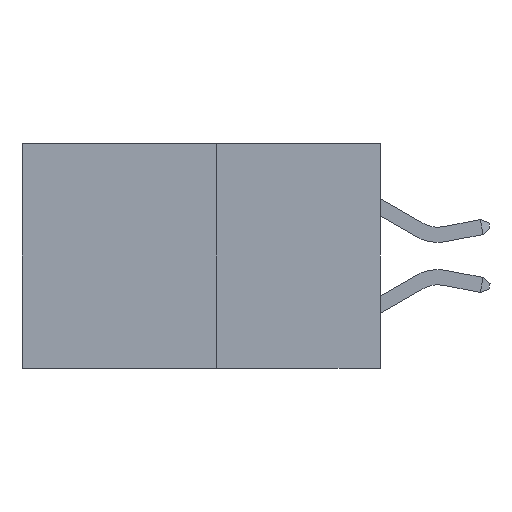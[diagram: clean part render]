
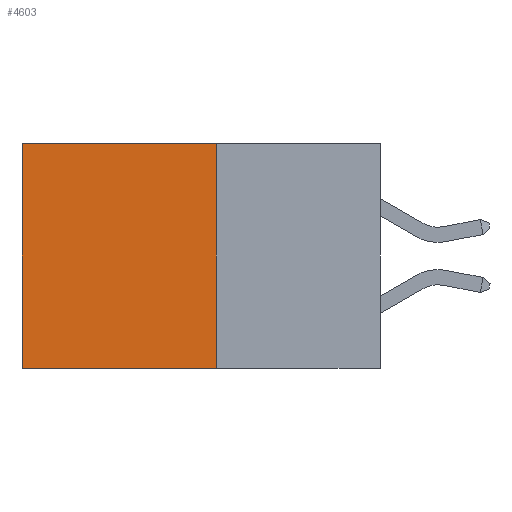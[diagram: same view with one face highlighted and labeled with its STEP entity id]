
A CAD part, left-side view. The second image highlights one B-rep face of the part: STEP entity #4603.
In plain terms, the highlighted planar face has unit normal (-1, 0, 0).
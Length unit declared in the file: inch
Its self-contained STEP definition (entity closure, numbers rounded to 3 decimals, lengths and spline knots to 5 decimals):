
#273 = FACE_OUTER_BOUND ( 'NONE', #3999, .T. ) ;
#633 = ORIENTED_EDGE ( 'NONE', *, *, #11598, .T. ) ;
#1055 = CARTESIAN_POINT ( 'NONE',  ( 0.277, 0.59, -0.37 ) ) ;
#1061 = LINE ( 'NONE', #1055, #3337 ) ;
#1220 = DIRECTION ( 'NONE',  ( 0., 1., 0. ) ) ;
#2282 = EDGE_CURVE ( 'NONE', #11697, #4051, #3701, .T. ) ;
#2410 = EDGE_CURVE ( 'NONE', #8951, #11697, #11382, .T. ) ;
#2413 = LINE ( 'NONE', #6944, #7732 ) ;
#3337 = VECTOR ( 'NONE', #11018, 39.37008 ) ;
#3382 = VECTOR ( 'NONE', #3425, 39.37008 ) ;
#3425 = DIRECTION ( 'NONE',  ( 0., 1., 0. ) ) ;
#3701 = LINE ( 'NONE', #7364, #3382 ) ;
#3999 = EDGE_LOOP ( 'NONE', ( #5461, #9014, #9781, #633 ) ) ;
#4051 = VERTEX_POINT ( 'NONE', #7187 ) ;
#4142 = VECTOR ( 'NONE', #9307, 39.37008 ) ;
#4603 = ADVANCED_FACE ( 'NONE', ( #273 ), #11090, .F. ) ;
#5461 = ORIENTED_EDGE ( 'NONE', *, *, #11503, .T. ) ;
#6927 = CARTESIAN_POINT ( 'NONE',  ( 0.277, 0.27, 0. ) ) ;
#6944 = CARTESIAN_POINT ( 'NONE',  ( 0.277, 0.27, 0. ) ) ;
#7187 = CARTESIAN_POINT ( 'NONE',  ( 0.277, 0.59, -0.37 ) ) ;
#7364 = CARTESIAN_POINT ( 'NONE',  ( 0.277, 0.27, -0.37 ) ) ;
#7732 = VECTOR ( 'NONE', #1220, 39.37008 ) ;
#8664 = DIRECTION ( 'NONE',  ( 1., 0., 0. ) ) ;
#8951 = VERTEX_POINT ( 'NONE', #6927 ) ;
#9014 = ORIENTED_EDGE ( 'NONE', *, *, #2282, .F. ) ;
#9307 = DIRECTION ( 'NONE',  ( 0., 0., -1. ) ) ;
#9651 = CARTESIAN_POINT ( 'NONE',  ( 0.277, 0.27, -0.37 ) ) ;
#9781 = ORIENTED_EDGE ( 'NONE', *, *, #2410, .F. ) ;
#9792 = AXIS2_PLACEMENT_3D ( 'NONE', #10401, #8664, #10765 ) ;
#9811 = CARTESIAN_POINT ( 'NONE',  ( 0.277, 0.27, -0.37 ) ) ;
#10361 = CARTESIAN_POINT ( 'NONE',  ( 0.277, 0.59, 0. ) ) ;
#10401 = CARTESIAN_POINT ( 'NONE',  ( 0.277, 0.27, -0.37 ) ) ;
#10765 = DIRECTION ( 'NONE',  ( 0., 0., -1. ) ) ;
#10951 = VERTEX_POINT ( 'NONE', #10361 ) ;
#11018 = DIRECTION ( 'NONE',  ( 0., 0., -1. ) ) ;
#11090 = PLANE ( 'NONE',  #9792 ) ;
#11382 = LINE ( 'NONE', #9811, #4142 ) ;
#11503 = EDGE_CURVE ( 'NONE', #10951, #4051, #1061, .T. ) ;
#11598 = EDGE_CURVE ( 'NONE', #8951, #10951, #2413, .T. ) ;
#11697 = VERTEX_POINT ( 'NONE', #9651 ) ;
